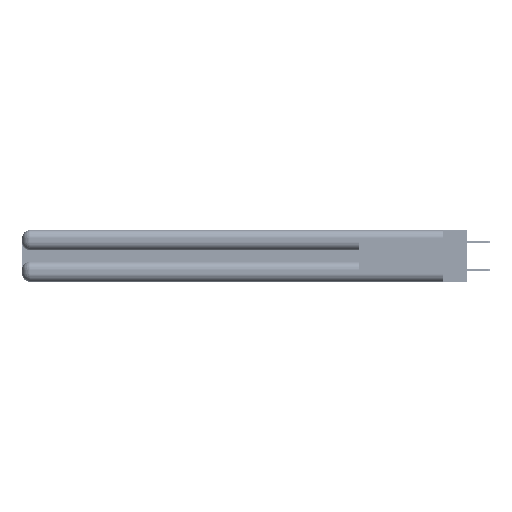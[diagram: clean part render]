
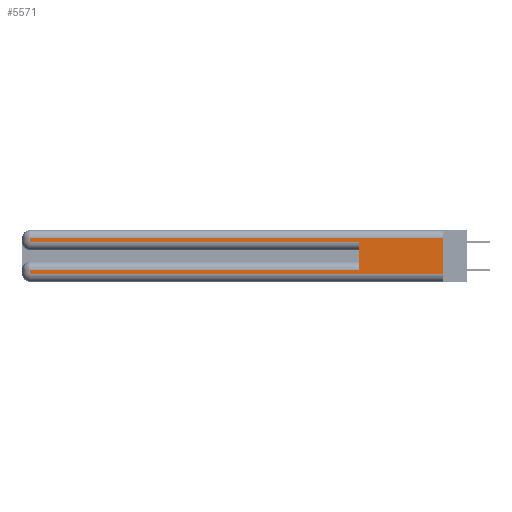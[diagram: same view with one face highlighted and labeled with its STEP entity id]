
A CAD part, left-side view. The second image highlights one B-rep face of the part: STEP entity #5571.
In plain terms, the highlighted planar face has unit normal (-1, 0, 0).
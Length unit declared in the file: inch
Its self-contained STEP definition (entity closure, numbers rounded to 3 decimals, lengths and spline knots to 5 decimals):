
#31 = VECTOR ( 'NONE', #7358, 39.37008 ) ;
#600 = DIRECTION ( 'NONE',  ( 0., -1., 0. ) ) ;
#1154 = VERTEX_POINT ( 'NONE', #43436 ) ;
#1640 = ORIENTED_EDGE ( 'NONE', *, *, #24232, .F. ) ;
#2959 = VERTEX_POINT ( 'NONE', #39943 ) ;
#4709 = CARTESIAN_POINT ( 'NONE',  ( 0., 0., 0.37 ) ) ;
#4714 = CARTESIAN_POINT ( 'NONE',  ( 0., 0., 0.06 ) ) ;
#5571 = ADVANCED_FACE ( 'NONE', ( #16195 ), #46092, .F. ) ;
#5636 = CARTESIAN_POINT ( 'NONE',  ( 0., 0.6, 0.285 ) ) ;
#5727 = VECTOR ( 'NONE', #600, 39.37008 ) ;
#6662 = LINE ( 'NONE', #4714, #35292 ) ;
#7358 = DIRECTION ( 'NONE',  ( 0., 0., -1. ) ) ;
#8812 = DIRECTION ( 'NONE',  ( 0., 0., -1. ) ) ;
#9229 = LINE ( 'NONE', #25009, #32734 ) ;
#11034 = DIRECTION ( 'NONE',  ( 0., 1., 0. ) ) ;
#12165 = ORIENTED_EDGE ( 'NONE', *, *, #52255, .T. ) ;
#14068 = ORIENTED_EDGE ( 'NONE', *, *, #15352, .F. ) ;
#14484 = LINE ( 'NONE', #32640, #27211 ) ;
#15352 = EDGE_CURVE ( 'NONE', #41908, #23565, #14484, .T. ) ;
#15367 = VECTOR ( 'NONE', #8812, 39.37008 ) ;
#16195 = FACE_OUTER_BOUND ( 'NONE', #23072, .T. ) ;
#16536 = LINE ( 'NONE', #45114, #28605 ) ;
#16834 = AXIS2_PLACEMENT_3D ( 'NONE', #17458, #22032, #41802 ) ;
#17139 = ORIENTED_EDGE ( 'NONE', *, *, #24892, .T. ) ;
#17204 = ORIENTED_EDGE ( 'NONE', *, *, #48061, .T. ) ;
#17458 = CARTESIAN_POINT ( 'NONE',  ( 0., 0., 0.37 ) ) ;
#17725 = CARTESIAN_POINT ( 'NONE',  ( 0., 2.94, 0.085 ) ) ;
#19728 = CARTESIAN_POINT ( 'NONE',  ( 0., 0., 0.31 ) ) ;
#19996 = CARTESIAN_POINT ( 'NONE',  ( 0., 0., 0.285 ) ) ;
#20145 = CARTESIAN_POINT ( 'NONE',  ( 0., 2.94, 0.285 ) ) ;
#20180 = DIRECTION ( 'NONE',  ( 0., 0., 1. ) ) ;
#21058 = VERTEX_POINT ( 'NONE', #25097 ) ;
#21483 = CARTESIAN_POINT ( 'NONE',  ( 0., 2.94, 0.31 ) ) ;
#22032 = DIRECTION ( 'NONE',  ( 1., 0., 0. ) ) ;
#23072 = EDGE_LOOP ( 'NONE', ( #1640, #17204, #12165, #47668, #14068, #51535, #17139, #45222 ) ) ;
#23565 = VERTEX_POINT ( 'NONE', #5636 ) ;
#24232 = EDGE_CURVE ( 'NONE', #2959, #1154, #40180, .T. ) ;
#24799 = LINE ( 'NONE', #27766, #31 ) ;
#24892 = EDGE_CURVE ( 'NONE', #40284, #21058, #16536, .T. ) ;
#25009 = CARTESIAN_POINT ( 'NONE',  ( 0., 0., 0.085 ) ) ;
#25097 = CARTESIAN_POINT ( 'NONE',  ( 0., 2.94, 0.06 ) ) ;
#25350 = CARTESIAN_POINT ( 'NONE',  ( 0., 0.6, 0.085 ) ) ;
#25490 = DIRECTION ( 'NONE',  ( 0., -1., 0. ) ) ;
#27211 = VECTOR ( 'NONE', #20180, 39.37008 ) ;
#27712 = VECTOR ( 'NONE', #11034, 39.37008 ) ;
#27766 = CARTESIAN_POINT ( 'NONE',  ( 0., 2.94, 0.37 ) ) ;
#28384 = DIRECTION ( 'NONE',  ( 0., 1., 0. ) ) ;
#28605 = VECTOR ( 'NONE', #37637, 39.37008 ) ;
#32640 = CARTESIAN_POINT ( 'NONE',  ( 0., 0.6, 0.145 ) ) ;
#32734 = VECTOR ( 'NONE', #28384, 39.37008 ) ;
#35292 = VECTOR ( 'NONE', #25490, 39.37008 ) ;
#35605 = VERTEX_POINT ( 'NONE', #20145 ) ;
#35641 = LINE ( 'NONE', #19996, #5727 ) ;
#36745 = LINE ( 'NONE', #19728, #27712 ) ;
#37637 = DIRECTION ( 'NONE',  ( 0., 0., -1. ) ) ;
#39144 = VERTEX_POINT ( 'NONE', #21483 ) ;
#39943 = CARTESIAN_POINT ( 'NONE',  ( 0., 0., 0.31 ) ) ;
#40180 = LINE ( 'NONE', #4709, #15367 ) ;
#40284 = VERTEX_POINT ( 'NONE', #17725 ) ;
#41802 = DIRECTION ( 'NONE',  ( 0., 0., -1. ) ) ;
#41908 = VERTEX_POINT ( 'NONE', #25350 ) ;
#43436 = CARTESIAN_POINT ( 'NONE',  ( 0., 0., 0.06 ) ) ;
#45114 = CARTESIAN_POINT ( 'NONE',  ( 0., 2.94, 0.37 ) ) ;
#45222 = ORIENTED_EDGE ( 'NONE', *, *, #46987, .T. ) ;
#46092 = PLANE ( 'NONE',  #16834 ) ;
#46987 = EDGE_CURVE ( 'NONE', #21058, #1154, #6662, .T. ) ;
#47668 = ORIENTED_EDGE ( 'NONE', *, *, #52269, .T. ) ;
#48061 = EDGE_CURVE ( 'NONE', #2959, #39144, #36745, .T. ) ;
#49717 = EDGE_CURVE ( 'NONE', #41908, #40284, #9229, .T. ) ;
#51535 = ORIENTED_EDGE ( 'NONE', *, *, #49717, .T. ) ;
#52255 = EDGE_CURVE ( 'NONE', #39144, #35605, #24799, .T. ) ;
#52269 = EDGE_CURVE ( 'NONE', #35605, #23565, #35641, .T. ) ;
